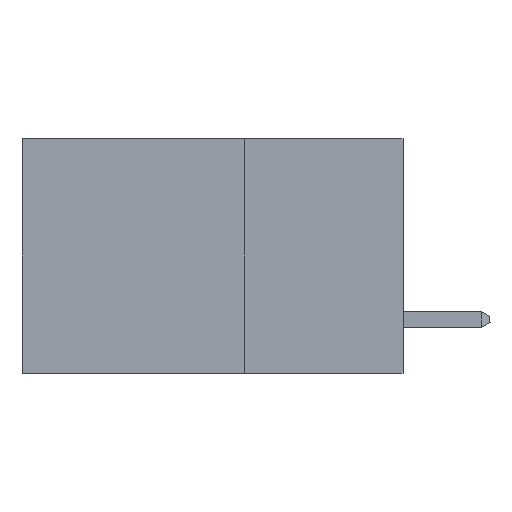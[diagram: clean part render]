
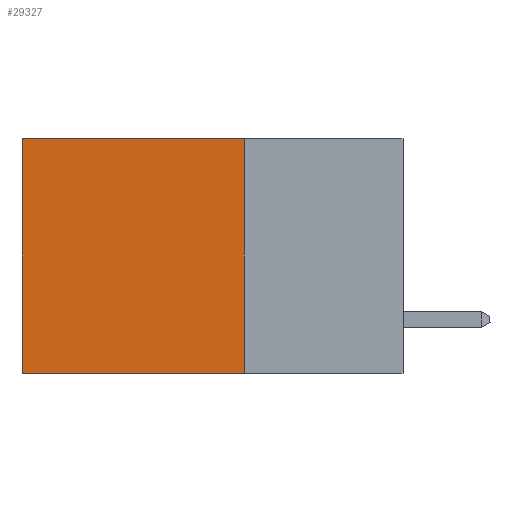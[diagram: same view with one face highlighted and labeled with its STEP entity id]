
A CAD part, left-side view. The second image highlights one B-rep face of the part: STEP entity #29327.
In plain terms, the highlighted planar face has unit normal (-1, 0, 0).
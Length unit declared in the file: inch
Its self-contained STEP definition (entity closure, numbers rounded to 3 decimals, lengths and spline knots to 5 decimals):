
#2497 = DIRECTION ( 'NONE',  ( 0., 0., -1. ) ) ;
#3356 = EDGE_CURVE ( 'NONE', #42834, #21805, #17314, .T. ) ;
#3958 = FACE_OUTER_BOUND ( 'NONE', #46625, .T. ) ;
#4404 = DIRECTION ( 'NONE',  ( 0., 0., -1. ) ) ;
#5629 = CARTESIAN_POINT ( 'NONE',  ( 0.2875, 0.25, -0.37 ) ) ;
#5921 = ORIENTED_EDGE ( 'NONE', *, *, #24269, .F. ) ;
#10104 = DIRECTION ( 'NONE',  ( 0., 1., 0. ) ) ;
#12061 = CARTESIAN_POINT ( 'NONE',  ( 0.2875, 0.25, 0. ) ) ;
#13164 = CARTESIAN_POINT ( 'NONE',  ( 0.2875, 0.25, -0.37 ) ) ;
#14566 = CARTESIAN_POINT ( 'NONE',  ( 0.2875, 0.6, 0. ) ) ;
#16122 = DIRECTION ( 'NONE',  ( 1., 0., 0. ) ) ;
#16196 = CARTESIAN_POINT ( 'NONE',  ( 0.2875, 0.6, 0. ) ) ;
#16949 = VERTEX_POINT ( 'NONE', #22768 ) ;
#17054 = CARTESIAN_POINT ( 'NONE',  ( 0.2875, 0.25, 0. ) ) ;
#17088 = LINE ( 'NONE', #5629, #19395 ) ;
#17314 = LINE ( 'NONE', #16196, #27613 ) ;
#17753 = EDGE_CURVE ( 'NONE', #23303, #21805, #17088, .T. ) ;
#18057 = EDGE_CURVE ( 'NONE', #16949, #42834, #40512, .T. ) ;
#18212 = AXIS2_PLACEMENT_3D ( 'NONE', #12061, #16122, #45620 ) ;
#19395 = VECTOR ( 'NONE', #28313, 39.37008 ) ;
#20268 = ORIENTED_EDGE ( 'NONE', *, *, #3356, .T. ) ;
#21532 = CARTESIAN_POINT ( 'NONE',  ( 0.2875, 0.6, -0.37 ) ) ;
#21805 = VERTEX_POINT ( 'NONE', #21532 ) ;
#22768 = CARTESIAN_POINT ( 'NONE',  ( 0.2875, 0.25, 0. ) ) ;
#23303 = VERTEX_POINT ( 'NONE', #13164 ) ;
#24269 = EDGE_CURVE ( 'NONE', #16949, #23303, #40707, .T. ) ;
#27613 = VECTOR ( 'NONE', #2497, 39.37008 ) ;
#28313 = DIRECTION ( 'NONE',  ( 0., 1., 0. ) ) ;
#29304 = VECTOR ( 'NONE', #4404, 39.37008 ) ;
#29327 = ADVANCED_FACE ( 'NONE', ( #3958 ), #33846, .F. ) ;
#33846 = PLANE ( 'NONE',  #18212 ) ;
#36816 = CARTESIAN_POINT ( 'NONE',  ( 0.2875, 0.25, 0. ) ) ;
#37033 = ORIENTED_EDGE ( 'NONE', *, *, #18057, .T. ) ;
#40512 = LINE ( 'NONE', #17054, #42256 ) ;
#40707 = LINE ( 'NONE', #36816, #29304 ) ;
#42256 = VECTOR ( 'NONE', #10104, 39.37008 ) ;
#42834 = VERTEX_POINT ( 'NONE', #14566 ) ;
#44404 = ORIENTED_EDGE ( 'NONE', *, *, #17753, .F. ) ;
#45620 = DIRECTION ( 'NONE',  ( 0., 0., -1. ) ) ;
#46625 = EDGE_LOOP ( 'NONE', ( #20268, #44404, #5921, #37033 ) ) ;
